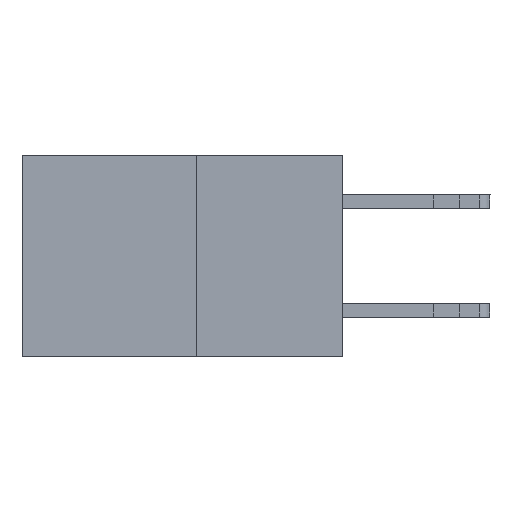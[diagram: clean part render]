
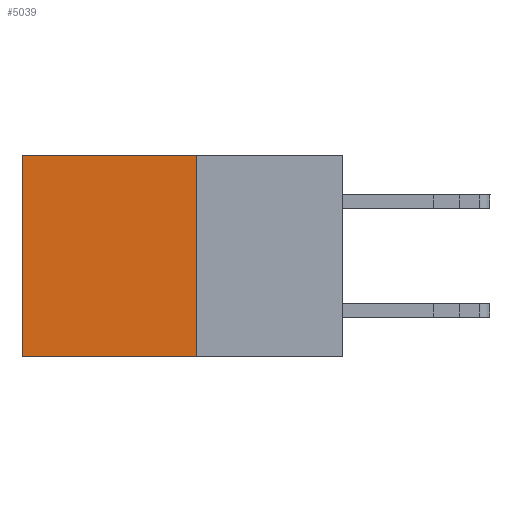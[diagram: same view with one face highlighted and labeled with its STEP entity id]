
A CAD part, left-side view. The second image highlights one B-rep face of the part: STEP entity #5039.
In plain terms, the highlighted planar face has unit normal (-1, 0, 0).
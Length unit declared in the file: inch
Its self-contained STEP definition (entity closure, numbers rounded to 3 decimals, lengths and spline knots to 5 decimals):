
#833 = DIRECTION ( 'NONE',  ( 0., 0., -1. ) ) ;
#1148 = VERTEX_POINT ( 'NONE', #8416 ) ;
#1224 = VECTOR ( 'NONE', #10167, 39.37008 ) ;
#1561 = EDGE_LOOP ( 'NONE', ( #7203, #12348, #12993, #3811 ) ) ;
#2166 = VECTOR ( 'NONE', #4589, 39.37008 ) ;
#3811 = ORIENTED_EDGE ( 'NONE', *, *, #13754, .T. ) ;
#3924 = CARTESIAN_POINT ( 'NONE',  ( 0.277, 0.27, -0.37 ) ) ;
#3964 = CARTESIAN_POINT ( 'NONE',  ( 0.277, 0.59, -0.37 ) ) ;
#4184 = LINE ( 'NONE', #12623, #4515 ) ;
#4210 = DIRECTION ( 'NONE',  ( 1., 0., 0. ) ) ;
#4515 = VECTOR ( 'NONE', #8464, 39.37008 ) ;
#4522 = LINE ( 'NONE', #12315, #2166 ) ;
#4589 = DIRECTION ( 'NONE',  ( 0., 0., -1. ) ) ;
#5039 = ADVANCED_FACE ( 'NONE', ( #9347 ), #8492, .F. ) ;
#5126 = VECTOR ( 'NONE', #5486, 39.37008 ) ;
#5486 = DIRECTION ( 'NONE',  ( 0., 1., 0. ) ) ;
#5649 = AXIS2_PLACEMENT_3D ( 'NONE', #13862, #4210, #833 ) ;
#6502 = VERTEX_POINT ( 'NONE', #12478 ) ;
#6626 = CARTESIAN_POINT ( 'NONE',  ( 0.277, 0.27, -0.37 ) ) ;
#7203 = ORIENTED_EDGE ( 'NONE', *, *, #7733, .T. ) ;
#7733 = EDGE_CURVE ( 'NONE', #12613, #6502, #9235, .T. ) ;
#8416 = CARTESIAN_POINT ( 'NONE',  ( 0.277, 0.27, 0. ) ) ;
#8464 = DIRECTION ( 'NONE',  ( 0., 1., 0. ) ) ;
#8492 = PLANE ( 'NONE',  #5649 ) ;
#8552 = EDGE_CURVE ( 'NONE', #8789, #6502, #9782, .T. ) ;
#8789 = VERTEX_POINT ( 'NONE', #3924 ) ;
#9235 = LINE ( 'NONE', #3964, #1224 ) ;
#9347 = FACE_OUTER_BOUND ( 'NONE', #1561, .T. ) ;
#9438 = EDGE_CURVE ( 'NONE', #1148, #8789, #4522, .T. ) ;
#9782 = LINE ( 'NONE', #6626, #5126 ) ;
#10167 = DIRECTION ( 'NONE',  ( 0., 0., -1. ) ) ;
#11083 = CARTESIAN_POINT ( 'NONE',  ( 0.277, 0.59, 0. ) ) ;
#12315 = CARTESIAN_POINT ( 'NONE',  ( 0.277, 0.27, -0.37 ) ) ;
#12348 = ORIENTED_EDGE ( 'NONE', *, *, #8552, .F. ) ;
#12478 = CARTESIAN_POINT ( 'NONE',  ( 0.277, 0.59, -0.37 ) ) ;
#12613 = VERTEX_POINT ( 'NONE', #11083 ) ;
#12623 = CARTESIAN_POINT ( 'NONE',  ( 0.277, 0.27, 0. ) ) ;
#12993 = ORIENTED_EDGE ( 'NONE', *, *, #9438, .F. ) ;
#13754 = EDGE_CURVE ( 'NONE', #1148, #12613, #4184, .T. ) ;
#13862 = CARTESIAN_POINT ( 'NONE',  ( 0.277, 0.27, -0.37 ) ) ;
